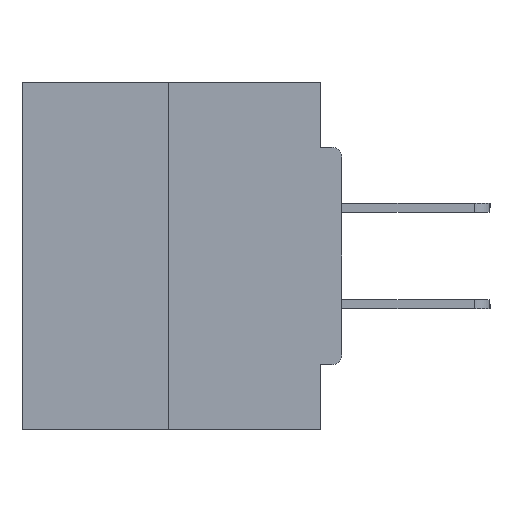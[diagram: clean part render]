
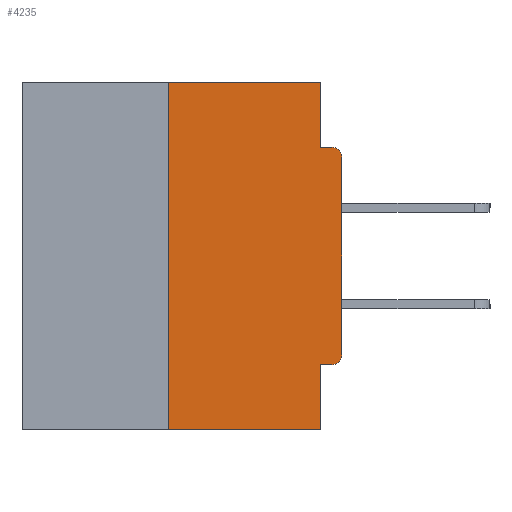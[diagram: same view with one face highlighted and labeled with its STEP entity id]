
A CAD part, left-side view. The second image highlights one B-rep face of the part: STEP entity #4235.
In plain terms, the highlighted planar face has unit normal (-1, 0, 0).
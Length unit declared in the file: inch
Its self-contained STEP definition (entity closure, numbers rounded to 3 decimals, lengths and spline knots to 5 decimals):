
#418 = DIRECTION ( 'NONE',  ( 0., 0., -1. ) ) ;
#1034 = CARTESIAN_POINT ( 'NONE',  ( 0., 0., -0.1085 ) ) ;
#1060 = VERTEX_POINT ( 'NONE', #3190 ) ;
#1189 = ORIENTED_EDGE ( 'NONE', *, *, #27194, .F. ) ;
#1757 = LINE ( 'NONE', #20823, #33565 ) ;
#1998 = CARTESIAN_POINT ( 'NONE',  ( 0., 0.031, -0.0935 ) ) ;
#2154 = CARTESIAN_POINT ( 'NONE',  ( 0., 0.46, 0. ) ) ;
#2170 = ORIENTED_EDGE ( 'NONE', *, *, #26125, .F. ) ;
#2522 = VECTOR ( 'NONE', #17940, 39.37008 ) ;
#3173 = EDGE_CURVE ( 'NONE', #9158, #16013, #24165, .T. ) ;
#3190 = CARTESIAN_POINT ( 'NONE',  ( 0., 0.031, 0. ) ) ;
#3299 = DIRECTION ( 'NONE',  ( 0., 0., -1. ) ) ;
#3737 = AXIS2_PLACEMENT_3D ( 'NONE', #33169, #28186, #22473 ) ;
#4051 = DIRECTION ( 'NONE',  ( 0., 0., 1. ) ) ;
#4092 = LINE ( 'NONE', #2154, #22049 ) ;
#4235 = ADVANCED_FACE ( 'NONE', ( #19434 ), #22285, .F. ) ;
#5943 = DIRECTION ( 'NONE',  ( -1., 0., 0. ) ) ;
#6789 = DIRECTION ( 'NONE',  ( 0., 0., -1. ) ) ;
#7790 = CARTESIAN_POINT ( 'NONE',  ( 0., 0.25, 0. ) ) ;
#7897 = EDGE_CURVE ( 'NONE', #9158, #35206, #13887, .T. ) ;
#9158 = VERTEX_POINT ( 'NONE', #12208 ) ;
#9394 = CIRCLE ( 'NONE', #29351, 0.015 ) ;
#9674 = CARTESIAN_POINT ( 'NONE',  ( 0., 0.015, -0.4065 ) ) ;
#9691 = ORIENTED_EDGE ( 'NONE', *, *, #34815, .F. ) ;
#10849 = EDGE_CURVE ( 'NONE', #19335, #23687, #14726, .T. ) ;
#11261 = CARTESIAN_POINT ( 'NONE',  ( 0., 0.015, -0.3915 ) ) ;
#11359 = EDGE_CURVE ( 'NONE', #23687, #15730, #34000, .T. ) ;
#11475 = ORIENTED_EDGE ( 'NONE', *, *, #11359, .T. ) ;
#11534 = CARTESIAN_POINT ( 'NONE',  ( 0., 0.46, -0.5 ) ) ;
#12208 = CARTESIAN_POINT ( 'NONE',  ( 0., 0.25, -0.5 ) ) ;
#12484 = ORIENTED_EDGE ( 'NONE', *, *, #28187, .F. ) ;
#12503 = CARTESIAN_POINT ( 'NONE',  ( 0., 0.015, -0.0935 ) ) ;
#13274 = VECTOR ( 'NONE', #3299, 39.37008 ) ;
#13821 = LINE ( 'NONE', #22544, #13274 ) ;
#13887 = LINE ( 'NONE', #11534, #21489 ) ;
#14726 = CIRCLE ( 'NONE', #30132, 0.015 ) ;
#15266 = CARTESIAN_POINT ( 'NONE',  ( 0., 0., -0.4065 ) ) ;
#15336 = EDGE_CURVE ( 'NONE', #15730, #30236, #9394, .T. ) ;
#15730 = VERTEX_POINT ( 'NONE', #1034 ) ;
#15773 = DIRECTION ( 'NONE',  ( 0., 0., 1. ) ) ;
#16013 = VERTEX_POINT ( 'NONE', #16148 ) ;
#16148 = CARTESIAN_POINT ( 'NONE',  ( 0., 0.25, 0. ) ) ;
#17940 = DIRECTION ( 'NONE',  ( 0., 1., 0. ) ) ;
#17989 = DIRECTION ( 'NONE',  ( 0., -1., 0. ) ) ;
#19335 = VERTEX_POINT ( 'NONE', #9674 ) ;
#19434 = FACE_OUTER_BOUND ( 'NONE', #25194, .T. ) ;
#20655 = DIRECTION ( 'NONE',  ( -1., 0., 0. ) ) ;
#20823 = CARTESIAN_POINT ( 'NONE',  ( 0., 0., -0.0935 ) ) ;
#21261 = CARTESIAN_POINT ( 'NONE',  ( 0., 0.031, -0.5 ) ) ;
#21489 = VECTOR ( 'NONE', #24569, 39.37008 ) ;
#21719 = EDGE_CURVE ( 'NONE', #16013, #1060, #4092, .T. ) ;
#21763 = ORIENTED_EDGE ( 'NONE', *, *, #3173, .F. ) ;
#22049 = VECTOR ( 'NONE', #17989, 39.37008 ) ;
#22285 = PLANE ( 'NONE',  #3737 ) ;
#22473 = DIRECTION ( 'NONE',  ( 0., 0., -1. ) ) ;
#22544 = CARTESIAN_POINT ( 'NONE',  ( 0., 0.031, 0. ) ) ;
#22914 = CARTESIAN_POINT ( 'NONE',  ( 0., 0.031, -0.4065 ) ) ;
#23309 = CARTESIAN_POINT ( 'NONE',  ( 0., 0., 0. ) ) ;
#23687 = VERTEX_POINT ( 'NONE', #27053 ) ;
#24165 = LINE ( 'NONE', #7790, #33859 ) ;
#24569 = DIRECTION ( 'NONE',  ( 0., -1., 0. ) ) ;
#24986 = VERTEX_POINT ( 'NONE', #1998 ) ;
#25194 = EDGE_LOOP ( 'NONE', ( #28982, #21763, #33598, #12484, #1189, #29419, #11475, #32231, #9691, #2170 ) ) ;
#26125 = EDGE_CURVE ( 'NONE', #1060, #24986, #13821, .T. ) ;
#26772 = CARTESIAN_POINT ( 'NONE',  ( 0., 0.031, -0.5 ) ) ;
#26945 = LINE ( 'NONE', #26772, #30481 ) ;
#27053 = CARTESIAN_POINT ( 'NONE',  ( 0., 0., -0.3915 ) ) ;
#27194 = EDGE_CURVE ( 'NONE', #19335, #31030, #31175, .T. ) ;
#28186 = DIRECTION ( 'NONE',  ( 1., 0., 0. ) ) ;
#28187 = EDGE_CURVE ( 'NONE', #31030, #35206, #26945, .T. ) ;
#28982 = ORIENTED_EDGE ( 'NONE', *, *, #21719, .F. ) ;
#29351 = AXIS2_PLACEMENT_3D ( 'NONE', #34559, #20655, #6789 ) ;
#29419 = ORIENTED_EDGE ( 'NONE', *, *, #10849, .T. ) ;
#30132 = AXIS2_PLACEMENT_3D ( 'NONE', #11261, #5943, #418 ) ;
#30236 = VERTEX_POINT ( 'NONE', #12503 ) ;
#30481 = VECTOR ( 'NONE', #31780, 39.37008 ) ;
#31030 = VERTEX_POINT ( 'NONE', #22914 ) ;
#31175 = LINE ( 'NONE', #15266, #2522 ) ;
#31780 = DIRECTION ( 'NONE',  ( 0., 0., -1. ) ) ;
#31886 = DIRECTION ( 'NONE',  ( 0., -1., 0. ) ) ;
#32231 = ORIENTED_EDGE ( 'NONE', *, *, #15336, .T. ) ;
#33169 = CARTESIAN_POINT ( 'NONE',  ( 0., 0.46, 0. ) ) ;
#33565 = VECTOR ( 'NONE', #31886, 39.37008 ) ;
#33598 = ORIENTED_EDGE ( 'NONE', *, *, #7897, .T. ) ;
#33859 = VECTOR ( 'NONE', #15773, 39.37008 ) ;
#34000 = LINE ( 'NONE', #23309, #34422 ) ;
#34422 = VECTOR ( 'NONE', #4051, 39.37008 ) ;
#34559 = CARTESIAN_POINT ( 'NONE',  ( 0., 0.015, -0.1085 ) ) ;
#34815 = EDGE_CURVE ( 'NONE', #24986, #30236, #1757, .T. ) ;
#35206 = VERTEX_POINT ( 'NONE', #21261 ) ;
